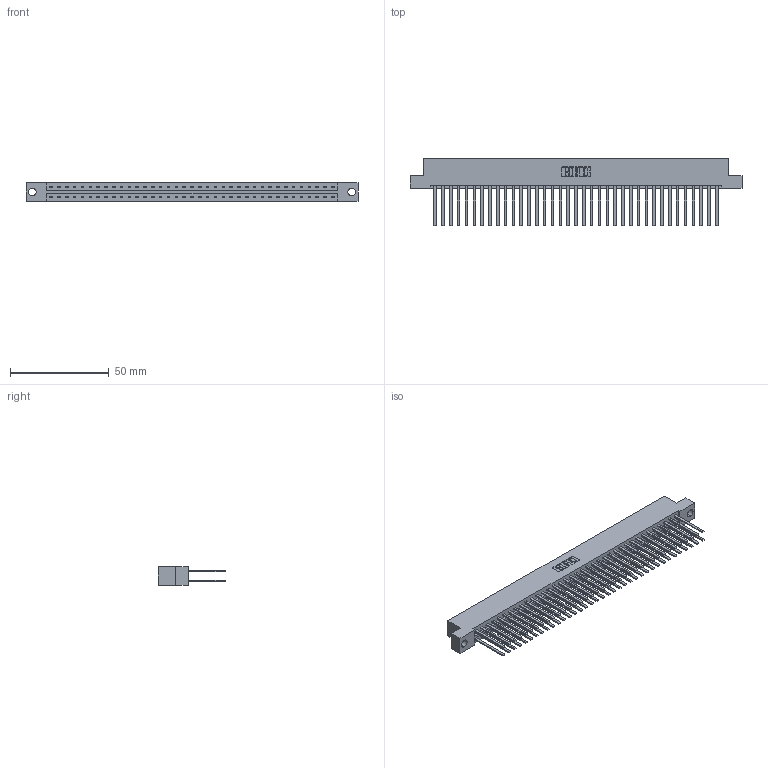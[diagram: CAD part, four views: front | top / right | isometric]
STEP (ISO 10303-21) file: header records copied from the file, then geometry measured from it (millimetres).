
FILE_DESCRIPTION (( 'STEP AP203' ), '1' );
FILE_NAME ('333-074-544-204.STEP', '2018-08-04T22:04:09', ( '' ), ( '' ), 'SwSTEP 2.0', 'SolidWorks 2016', '' );
FILE_SCHEMA (( 'CONFIG_CONTROL_DESIGN' ));
Length unit declared in the file: inch
Products named in the file (3): 333 Part_Flush - .156 Dia - TH; 345-292-001_345-293-144; 333-074-544-204
Assembly tree (75 placements, depth 2):
  333-074-544-204
    333 Part_Flush - .156 Dia - TH
    345-292-001_345-293-144  x74
Bounding box: 168.15 x 34.3 x 9.4 mm (x, y, z)
Volume: 18069.7 mm3; surface area: 24448.5 mm2
Topology: 75 solids, 75 shells, 3518 faces, 10449 edges, 6866 vertices
Faces by surface type: plane 2438, cylinder 1080
Entity records: 24269 total; most frequent: CARTESIAN_POINT 4026, ORIENTED_EDGE 3962, DIRECTION 3445, EDGE_CURVE 1981, VECTOR 1857, LINE 1857, VERTEX_POINT 1318, AXIS2_PLACEMENT_3D 794
